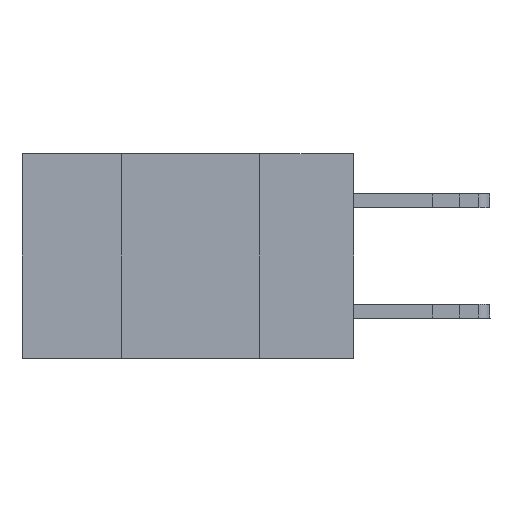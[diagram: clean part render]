
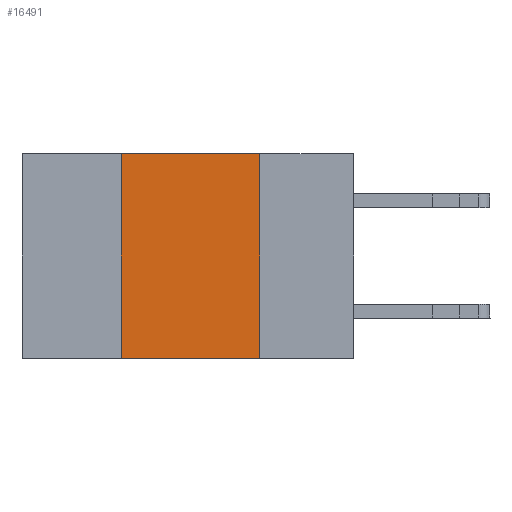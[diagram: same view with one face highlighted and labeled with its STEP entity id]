
A CAD part, left-side view. The second image highlights one B-rep face of the part: STEP entity #16491.
In plain terms, the highlighted planar face has unit normal (-1, 0, 0).
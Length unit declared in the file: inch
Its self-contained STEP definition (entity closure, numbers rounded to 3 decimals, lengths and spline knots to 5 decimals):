
#58 = VECTOR ( 'NONE', #2088, 39.37008 ) ;
#382 = CARTESIAN_POINT ( 'NONE',  ( 0., 0.42, -0.37 ) ) ;
#2012 = CARTESIAN_POINT ( 'NONE',  ( 0., 0.17, -0.37 ) ) ;
#2088 = DIRECTION ( 'NONE',  ( 0., -1., 0. ) ) ;
#2280 = AXIS2_PLACEMENT_3D ( 'NONE', #8768, #10651, #23483 ) ;
#5402 = CARTESIAN_POINT ( 'NONE',  ( 0., 0.6, -0.37 ) ) ;
#7441 = ORIENTED_EDGE ( 'NONE', *, *, #11576, .F. ) ;
#7465 = ORIENTED_EDGE ( 'NONE', *, *, #8992, .F. ) ;
#7488 = ORIENTED_EDGE ( 'NONE', *, *, #21052, .T. ) ;
#8389 = DIRECTION ( 'NONE',  ( 0., 0., -1. ) ) ;
#8768 = CARTESIAN_POINT ( 'NONE',  ( 0., 0.6, 0. ) ) ;
#8921 = VECTOR ( 'NONE', #8389, 39.37008 ) ;
#8949 = ORIENTED_EDGE ( 'NONE', *, *, #12258, .F. ) ;
#8992 = EDGE_CURVE ( 'NONE', #16328, #20186, #15304, .T. ) ;
#10651 = DIRECTION ( 'NONE',  ( 1., 0., 0. ) ) ;
#11576 = EDGE_CURVE ( 'NONE', #20186, #19214, #20253, .T. ) ;
#12258 = EDGE_CURVE ( 'NONE', #19214, #16834, #23008, .T. ) ;
#14096 = LINE ( 'NONE', #5402, #23305 ) ;
#14768 = DIRECTION ( 'NONE',  ( 0., -1., 0. ) ) ;
#15304 = LINE ( 'NONE', #23064, #23905 ) ;
#15736 = CARTESIAN_POINT ( 'NONE',  ( 0., 0.17, 0. ) ) ;
#16112 = PLANE ( 'NONE',  #2280 ) ;
#16328 = VERTEX_POINT ( 'NONE', #382 ) ;
#16491 = ADVANCED_FACE ( 'NONE', ( #22647 ), #16112, .F. ) ;
#16834 = VERTEX_POINT ( 'NONE', #2012 ) ;
#16845 = EDGE_LOOP ( 'NONE', ( #8949, #7441, #7465, #7488 ) ) ;
#17276 = CARTESIAN_POINT ( 'NONE',  ( 0., 0.6, 0. ) ) ;
#19214 = VERTEX_POINT ( 'NONE', #22062 ) ;
#20186 = VERTEX_POINT ( 'NONE', #21552 ) ;
#20253 = LINE ( 'NONE', #17276, #58 ) ;
#21052 = EDGE_CURVE ( 'NONE', #16328, #16834, #14096, .T. ) ;
#21552 = CARTESIAN_POINT ( 'NONE',  ( 0., 0.42, 0. ) ) ;
#22062 = CARTESIAN_POINT ( 'NONE',  ( 0., 0.17, 0. ) ) ;
#22647 = FACE_OUTER_BOUND ( 'NONE', #16845, .T. ) ;
#22987 = DIRECTION ( 'NONE',  ( 0., 0., 1. ) ) ;
#23008 = LINE ( 'NONE', #15736, #8921 ) ;
#23064 = CARTESIAN_POINT ( 'NONE',  ( 0., 0.42, 0. ) ) ;
#23305 = VECTOR ( 'NONE', #14768, 39.37008 ) ;
#23483 = DIRECTION ( 'NONE',  ( 0., 0., -1. ) ) ;
#23905 = VECTOR ( 'NONE', #22987, 39.37008 ) ;
